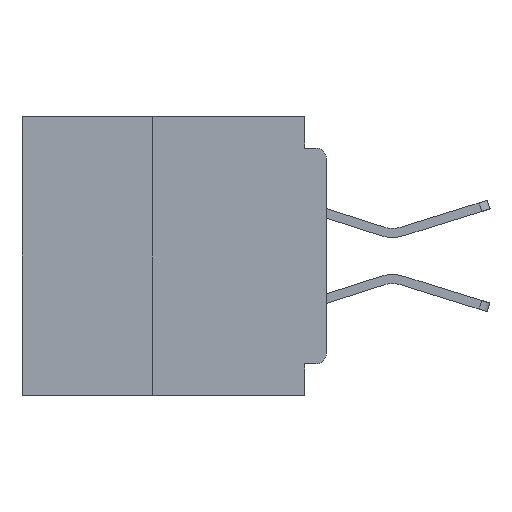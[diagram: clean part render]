
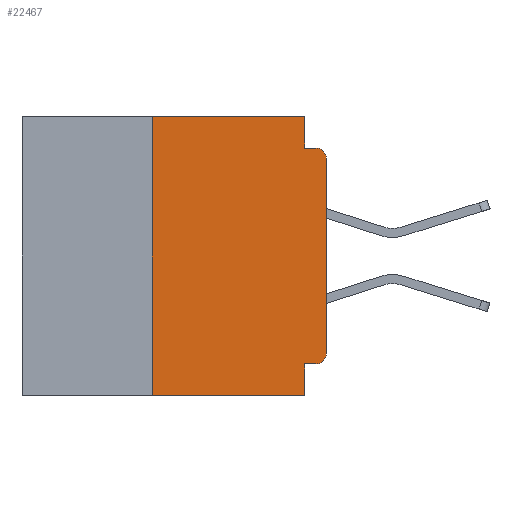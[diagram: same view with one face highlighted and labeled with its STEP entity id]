
A CAD part, left-side view. The second image highlights one B-rep face of the part: STEP entity #22467.
In plain terms, the highlighted planar face has unit normal (-1, 0, 0).
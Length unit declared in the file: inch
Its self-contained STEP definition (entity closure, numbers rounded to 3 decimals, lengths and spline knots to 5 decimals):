
#961 = VERTEX_POINT ( 'NONE', #52126 ) ;
#2350 = VECTOR ( 'NONE', #15399, 39.37008 ) ;
#2525 = DIRECTION ( 'NONE',  ( 0., 0., -1. ) ) ;
#3624 = VERTEX_POINT ( 'NONE', #6317 ) ;
#3834 = ORIENTED_EDGE ( 'NONE', *, *, #39334, .F. ) ;
#4582 = ORIENTED_EDGE ( 'NONE', *, *, #12223, .F. ) ;
#5461 = LINE ( 'NONE', #56462, #17646 ) ;
#6113 = EDGE_CURVE ( 'NONE', #41801, #22676, #21445, .T. ) ;
#6317 = CARTESIAN_POINT ( 'NONE',  ( 0., 0.015, -0.355 ) ) ;
#7590 = CARTESIAN_POINT ( 'NONE',  ( 0., 0.031, -0.4 ) ) ;
#7608 = ORIENTED_EDGE ( 'NONE', *, *, #6113, .T. ) ;
#7875 = VECTOR ( 'NONE', #29427, 39.37008 ) ;
#11836 = CARTESIAN_POINT ( 'NONE',  ( 0., 0.25, -0.4 ) ) ;
#12223 = EDGE_CURVE ( 'NONE', #961, #16574, #5461, .T. ) ;
#12893 = LINE ( 'NONE', #25897, #25012 ) ;
#14054 = CARTESIAN_POINT ( 'NONE',  ( 0., 0.25, -0.4 ) ) ;
#14059 = EDGE_CURVE ( 'NONE', #38985, #38840, #14533, .T. ) ;
#14533 = LINE ( 'NONE', #28895, #2350 ) ;
#15399 = DIRECTION ( 'NONE',  ( 0., 0., -1. ) ) ;
#15591 = AXIS2_PLACEMENT_3D ( 'NONE', #57014, #29833, #2525 ) ;
#15602 = DIRECTION ( 'NONE',  ( 0., 0., -1. ) ) ;
#16325 = VERTEX_POINT ( 'NONE', #37661 ) ;
#16574 = VERTEX_POINT ( 'NONE', #43786 ) ;
#17216 = CARTESIAN_POINT ( 'NONE',  ( 0., 0., -0.34 ) ) ;
#17646 = VECTOR ( 'NONE', #15602, 39.37008 ) ;
#17806 = CARTESIAN_POINT ( 'NONE',  ( 0., 0.015, -0.34 ) ) ;
#18767 = ORIENTED_EDGE ( 'NONE', *, *, #20216, .T. ) ;
#19045 = CARTESIAN_POINT ( 'NONE',  ( 0., 0.437, 0. ) ) ;
#20130 = CARTESIAN_POINT ( 'NONE',  ( 0., 0., -0.045 ) ) ;
#20216 = EDGE_CURVE ( 'NONE', #38295, #38840, #22840, .T. ) ;
#20741 = VECTOR ( 'NONE', #41277, 39.37008 ) ;
#21445 = LINE ( 'NONE', #52307, #7875 ) ;
#22361 = DIRECTION ( 'NONE',  ( 0., 0., -1. ) ) ;
#22467 = ADVANCED_FACE ( 'NONE', ( #26186 ), #48709, .F. ) ;
#22676 = VERTEX_POINT ( 'NONE', #58708 ) ;
#22840 = LINE ( 'NONE', #45110, #33451 ) ;
#23033 = VECTOR ( 'NONE', #46458, 39.37008 ) ;
#25012 = VECTOR ( 'NONE', #53075, 39.37008 ) ;
#25897 = CARTESIAN_POINT ( 'NONE',  ( 0., 0., -0.355 ) ) ;
#26055 = DIRECTION ( 'NONE',  ( 0., 0., -1. ) ) ;
#26186 = FACE_OUTER_BOUND ( 'NONE', #30483, .T. ) ;
#28657 = EDGE_CURVE ( 'NONE', #3624, #38985, #12893, .T. ) ;
#28726 = AXIS2_PLACEMENT_3D ( 'NONE', #44116, #53243, #26055 ) ;
#28895 = CARTESIAN_POINT ( 'NONE',  ( 0., 0.031, -0.4 ) ) ;
#29427 = DIRECTION ( 'NONE',  ( 0., 0., 1. ) ) ;
#29833 = DIRECTION ( 'NONE',  ( -1., 0., 0. ) ) ;
#30483 = EDGE_LOOP ( 'NONE', ( #7608, #43590, #3834, #4582, #40023, #42415, #18767, #31959, #34444, #45456 ) ) ;
#31227 = CARTESIAN_POINT ( 'NONE',  ( 0., 0.031, -0.355 ) ) ;
#31959 = ORIENTED_EDGE ( 'NONE', *, *, #14059, .F. ) ;
#33451 = VECTOR ( 'NONE', #36140, 39.37008 ) ;
#34086 = CIRCLE ( 'NONE', #52397, 0.015 ) ;
#34444 = ORIENTED_EDGE ( 'NONE', *, *, #28657, .F. ) ;
#35096 = LINE ( 'NONE', #19045, #23033 ) ;
#36140 = DIRECTION ( 'NONE',  ( 0., -1., 0. ) ) ;
#37661 = CARTESIAN_POINT ( 'NONE',  ( 0., 0.25, 0. ) ) ;
#38295 = VERTEX_POINT ( 'NONE', #11836 ) ;
#38356 = DIRECTION ( 'NONE',  ( 0., -1., 0. ) ) ;
#38812 = VERTEX_POINT ( 'NONE', #48384 ) ;
#38840 = VERTEX_POINT ( 'NONE', #7590 ) ;
#38985 = VERTEX_POINT ( 'NONE', #31227 ) ;
#39334 = EDGE_CURVE ( 'NONE', #16574, #38812, #41140, .T. ) ;
#40023 = ORIENTED_EDGE ( 'NONE', *, *, #53838, .F. ) ;
#41140 = LINE ( 'NONE', #20130, #51838 ) ;
#41277 = DIRECTION ( 'NONE',  ( 0., 0., 1. ) ) ;
#41801 = VERTEX_POINT ( 'NONE', #17216 ) ;
#42415 = ORIENTED_EDGE ( 'NONE', *, *, #44014, .F. ) ;
#43458 = LINE ( 'NONE', #14054, #20741 ) ;
#43590 = ORIENTED_EDGE ( 'NONE', *, *, #44955, .T. ) ;
#43786 = CARTESIAN_POINT ( 'NONE',  ( 0., 0.031, -0.045 ) ) ;
#44014 = EDGE_CURVE ( 'NONE', #38295, #16325, #43458, .T. ) ;
#44116 = CARTESIAN_POINT ( 'NONE',  ( 0., 0.437, 0. ) ) ;
#44955 = EDGE_CURVE ( 'NONE', #22676, #38812, #51190, .T. ) ;
#45110 = CARTESIAN_POINT ( 'NONE',  ( 0., 0.437, -0.4 ) ) ;
#45456 = ORIENTED_EDGE ( 'NONE', *, *, #48925, .T. ) ;
#46458 = DIRECTION ( 'NONE',  ( 0., -1., 0. ) ) ;
#48384 = CARTESIAN_POINT ( 'NONE',  ( 0., 0.015, -0.045 ) ) ;
#48709 = PLANE ( 'NONE',  #28726 ) ;
#48925 = EDGE_CURVE ( 'NONE', #3624, #41801, #34086, .T. ) ;
#49607 = DIRECTION ( 'NONE',  ( -1., 0., 0. ) ) ;
#51190 = CIRCLE ( 'NONE', #15591, 0.015 ) ;
#51838 = VECTOR ( 'NONE', #38356, 39.37008 ) ;
#52126 = CARTESIAN_POINT ( 'NONE',  ( 0., 0.031, 0. ) ) ;
#52307 = CARTESIAN_POINT ( 'NONE',  ( 0., 0., 0. ) ) ;
#52397 = AXIS2_PLACEMENT_3D ( 'NONE', #17806, #49607, #22361 ) ;
#53075 = DIRECTION ( 'NONE',  ( 0., 1., 0. ) ) ;
#53243 = DIRECTION ( 'NONE',  ( 1., 0., 0. ) ) ;
#53838 = EDGE_CURVE ( 'NONE', #16325, #961, #35096, .T. ) ;
#56462 = CARTESIAN_POINT ( 'NONE',  ( 0., 0.031, 0. ) ) ;
#57014 = CARTESIAN_POINT ( 'NONE',  ( 0., 0.015, -0.06 ) ) ;
#58708 = CARTESIAN_POINT ( 'NONE',  ( 0., 0., -0.06 ) ) ;
